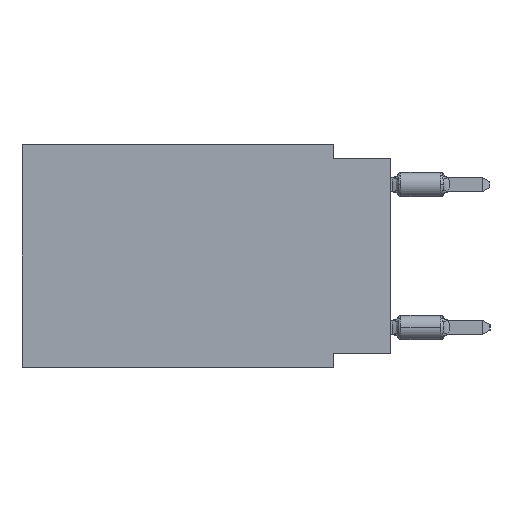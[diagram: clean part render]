
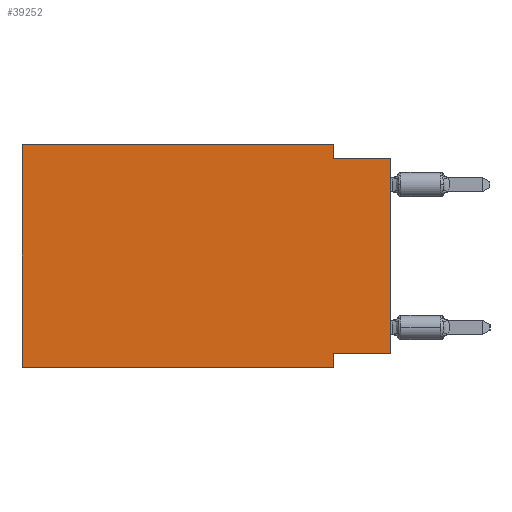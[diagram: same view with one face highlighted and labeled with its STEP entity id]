
A CAD part, left-side view. The second image highlights one B-rep face of the part: STEP entity #39252.
In plain terms, the highlighted planar face has unit normal (-1, 0, 0).
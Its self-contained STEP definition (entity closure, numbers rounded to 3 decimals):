
#46 = LINE ( 'NONE', #28238, #33959 ) ;
#2387 = VERTEX_POINT ( 'NONE', #38980 ) ;
#4282 = DIRECTION ( 'NONE',  ( 0., -1., 0. ) ) ;
#4479 = EDGE_CURVE ( 'NONE', #7778, #20296, #14445, .T. ) ;
#4733 = EDGE_CURVE ( 'NONE', #43483, #7709, #46, .T. ) ;
#5657 = DIRECTION ( 'NONE',  ( 0., 1., 0. ) ) ;
#5910 = DIRECTION ( 'NONE',  ( 0., -1., 0. ) ) ;
#7709 = VERTEX_POINT ( 'NONE', #49788 ) ;
#7778 = VERTEX_POINT ( 'NONE', #50600 ) ;
#8494 = CARTESIAN_POINT ( 'NONE',  ( 0., 16.383, -9.906 ) ) ;
#9434 = CARTESIAN_POINT ( 'NONE',  ( 0., 16.383, 0. ) ) ;
#10712 = DIRECTION ( 'NONE',  ( 1., 0., 0. ) ) ;
#11095 = CARTESIAN_POINT ( 'NONE',  ( 0., 0., -0.635 ) ) ;
#11146 = VECTOR ( 'NONE', #5910, 1000. ) ;
#12176 = ORIENTED_EDGE ( 'NONE', *, *, #4733, .F. ) ;
#12936 = ORIENTED_EDGE ( 'NONE', *, *, #4479, .F. ) ;
#14445 = LINE ( 'NONE', #47255, #39973 ) ;
#17054 = VECTOR ( 'NONE', #4282, 1000. ) ;
#17059 = CARTESIAN_POINT ( 'NONE',  ( 0., 0., -9.271 ) ) ;
#18400 = EDGE_CURVE ( 'NONE', #48750, #31084, #52845, .T. ) ;
#20296 = VERTEX_POINT ( 'NONE', #26695 ) ;
#21865 = FACE_OUTER_BOUND ( 'NONE', #41966, .T. ) ;
#22391 = DIRECTION ( 'NONE',  ( 0., 0., -1. ) ) ;
#22977 = CARTESIAN_POINT ( 'NONE',  ( 0., 0., -0.635 ) ) ;
#25208 = ORIENTED_EDGE ( 'NONE', *, *, #39983, .F. ) ;
#26629 = CARTESIAN_POINT ( 'NONE',  ( 0., 0., 0. ) ) ;
#26695 = CARTESIAN_POINT ( 'NONE',  ( 0., 2.54, -0.635 ) ) ;
#26775 = DIRECTION ( 'NONE',  ( 0., -1., 0. ) ) ;
#26992 = ORIENTED_EDGE ( 'NONE', *, *, #50850, .T. ) ;
#27410 = VECTOR ( 'NONE', #26775, 1000. ) ;
#28204 = ORIENTED_EDGE ( 'NONE', *, *, #37670, .F. ) ;
#28238 = CARTESIAN_POINT ( 'NONE',  ( 0., 16.383, 0. ) ) ;
#28878 = EDGE_CURVE ( 'NONE', #2387, #48238, #31486, .T. ) ;
#30029 = LINE ( 'NONE', #50931, #11146 ) ;
#31084 = VERTEX_POINT ( 'NONE', #52558 ) ;
#31486 = LINE ( 'NONE', #26629, #52685 ) ;
#33663 = VECTOR ( 'NONE', #5657, 1000. ) ;
#33958 = CARTESIAN_POINT ( 'NONE',  ( 0., 2.54, -9.271 ) ) ;
#33959 = VECTOR ( 'NONE', #37186, 1000. ) ;
#34574 = PLANE ( 'NONE',  #52657 ) ;
#35043 = DIRECTION ( 'NONE',  ( 0., 0., -1. ) ) ;
#35376 = CARTESIAN_POINT ( 'NONE',  ( 0., 16.383, 0. ) ) ;
#35567 = VECTOR ( 'NONE', #53110, 1000. ) ;
#36199 = ORIENTED_EDGE ( 'NONE', *, *, #18400, .F. ) ;
#37186 = DIRECTION ( 'NONE',  ( 0., 0., 1. ) ) ;
#37670 = EDGE_CURVE ( 'NONE', #20296, #48238, #38983, .T. ) ;
#38980 = CARTESIAN_POINT ( 'NONE',  ( 0., 0., -9.271 ) ) ;
#38983 = LINE ( 'NONE', #22977, #27410 ) ;
#39252 = ADVANCED_FACE ( 'NONE', ( #21865 ), #34574, .F. ) ;
#39973 = VECTOR ( 'NONE', #35043, 1000. ) ;
#39983 = EDGE_CURVE ( 'NONE', #2387, #48750, #45789, .T. ) ;
#41421 = LINE ( 'NONE', #9434, #17054 ) ;
#41966 = EDGE_LOOP ( 'NONE', ( #50362, #28204, #12936, #51050, #12176, #26992, #36199, #25208 ) ) ;
#43483 = VERTEX_POINT ( 'NONE', #8494 ) ;
#45789 = LINE ( 'NONE', #17059, #33663 ) ;
#46778 = EDGE_CURVE ( 'NONE', #7709, #7778, #41421, .T. ) ;
#47255 = CARTESIAN_POINT ( 'NONE',  ( 0., 2.54, 0. ) ) ;
#47503 = DIRECTION ( 'NONE',  ( 0., 0., 1. ) ) ;
#48238 = VERTEX_POINT ( 'NONE', #11095 ) ;
#48750 = VERTEX_POINT ( 'NONE', #33958 ) ;
#49788 = CARTESIAN_POINT ( 'NONE',  ( 0., 16.383, 0. ) ) ;
#50362 = ORIENTED_EDGE ( 'NONE', *, *, #28878, .T. ) ;
#50600 = CARTESIAN_POINT ( 'NONE',  ( 0., 2.54, 0. ) ) ;
#50850 = EDGE_CURVE ( 'NONE', #43483, #31084, #30029, .T. ) ;
#50931 = CARTESIAN_POINT ( 'NONE',  ( 0., 16.383, -9.906 ) ) ;
#51050 = ORIENTED_EDGE ( 'NONE', *, *, #46778, .F. ) ;
#52558 = CARTESIAN_POINT ( 'NONE',  ( 0., 2.54, -9.906 ) ) ;
#52657 = AXIS2_PLACEMENT_3D ( 'NONE', #35376, #10712, #22391 ) ;
#52685 = VECTOR ( 'NONE', #47503, 1000. ) ;
#52845 = LINE ( 'NONE', #53365, #35567 ) ;
#53110 = DIRECTION ( 'NONE',  ( 0., 0., -1. ) ) ;
#53365 = CARTESIAN_POINT ( 'NONE',  ( 0., 2.54, -9.906 ) ) ;
